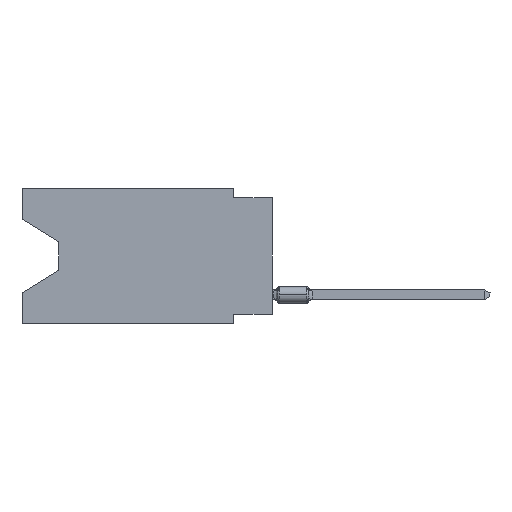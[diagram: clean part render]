
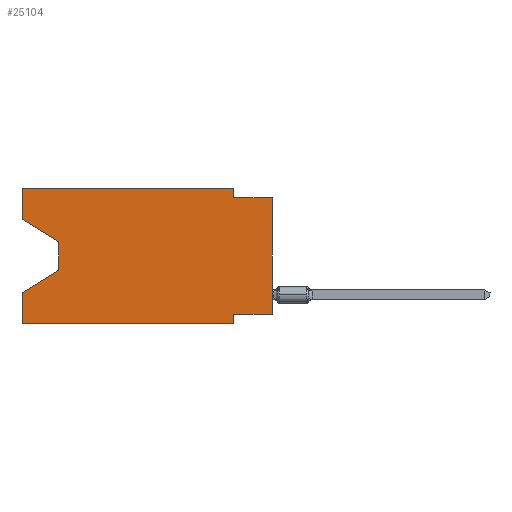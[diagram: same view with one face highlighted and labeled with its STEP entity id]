
A CAD part, left-side view. The second image highlights one B-rep face of the part: STEP entity #25104.
In plain terms, the highlighted planar face has unit normal (-1, 0, 0).
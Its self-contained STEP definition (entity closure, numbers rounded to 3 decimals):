
#1437 = VECTOR ( 'NONE', #28765, 1000. ) ;
#1544 = CARTESIAN_POINT ( 'NONE',  ( 0., 2.54, -0.635 ) ) ;
#2303 = CARTESIAN_POINT ( 'NONE',  ( 0., 2.54, -8.255 ) ) ;
#3989 = VECTOR ( 'NONE', #15168, 1000. ) ;
#4202 = VECTOR ( 'NONE', #17636, 1000. ) ;
#5450 = CARTESIAN_POINT ( 'NONE',  ( 0., 2.54, 0. ) ) ;
#5842 = VECTOR ( 'NONE', #18117, 1000. ) ;
#6163 = CARTESIAN_POINT ( 'NONE',  ( 0., 0., 0. ) ) ;
#6278 = VERTEX_POINT ( 'NONE', #1544 ) ;
#6721 = VERTEX_POINT ( 'NONE', #60788 ) ;
#7199 = EDGE_CURVE ( 'NONE', #6278, #15779, #60064, .T. ) ;
#8100 = ORIENTED_EDGE ( 'NONE', *, *, #58102, .T. ) ;
#9651 = VERTEX_POINT ( 'NONE', #30792 ) ;
#9822 = CARTESIAN_POINT ( 'NONE',  ( 0., 13.97, -3.505 ) ) ;
#9912 = ORIENTED_EDGE ( 'NONE', *, *, #25483, .T. ) ;
#10925 = LINE ( 'NONE', #55496, #21906 ) ;
#13155 = CARTESIAN_POINT ( 'NONE',  ( 0., 0., -0.635 ) ) ;
#14030 = CARTESIAN_POINT ( 'NONE',  ( 0., 13.97, -3.505 ) ) ;
#14526 = LINE ( 'NONE', #54491, #42638 ) ;
#14677 = DIRECTION ( 'NONE',  ( 0., 0., -1. ) ) ;
#15168 = DIRECTION ( 'NONE',  ( 0., -1., 0. ) ) ;
#15779 = VERTEX_POINT ( 'NONE', #13155 ) ;
#15805 = VERTEX_POINT ( 'NONE', #2303 ) ;
#17453 = CARTESIAN_POINT ( 'NONE',  ( 0., 13.97, -5.385 ) ) ;
#17636 = DIRECTION ( 'NONE',  ( 0., 0., 1. ) ) ;
#18117 = DIRECTION ( 'NONE',  ( 0., 0., -1. ) ) ;
#18408 = CARTESIAN_POINT ( 'NONE',  ( 0., 0., -8.255 ) ) ;
#19439 = DIRECTION ( 'NONE',  ( 0., -1., 0. ) ) ;
#20401 = VERTEX_POINT ( 'NONE', #29723 ) ;
#21127 = CARTESIAN_POINT ( 'NONE',  ( 0., 16.383, -6.852 ) ) ;
#21839 = VECTOR ( 'NONE', #31469, 1000. ) ;
#21906 = VECTOR ( 'NONE', #50893, 1000. ) ;
#22044 = LINE ( 'NONE', #17453, #44142 ) ;
#22450 = ORIENTED_EDGE ( 'NONE', *, *, #64841, .F. ) ;
#23852 = LINE ( 'NONE', #14030, #1437 ) ;
#23878 = VECTOR ( 'NONE', #45127, 1000. ) ;
#24247 = DIRECTION ( 'NONE',  ( 1., 0., 0. ) ) ;
#25104 = ADVANCED_FACE ( 'NONE', ( #58991 ), #54069, .F. ) ;
#25450 = EDGE_LOOP ( 'NONE', ( #8100, #9912, #36545, #36040, #64268, #38362, #22450, #37589, #34836, #39675, #56191, #43249 ) ) ;
#25483 = EDGE_CURVE ( 'NONE', #29320, #47591, #23852, .T. ) ;
#26862 = LINE ( 'NONE', #45880, #21839 ) ;
#27901 = EDGE_CURVE ( 'NONE', #46920, #57472, #14526, .T. ) ;
#28765 = DIRECTION ( 'NONE',  ( 0., 0., -1. ) ) ;
#29320 = VERTEX_POINT ( 'NONE', #9822 ) ;
#29723 = CARTESIAN_POINT ( 'NONE',  ( 0., 16.383, -2.038 ) ) ;
#30050 = EDGE_CURVE ( 'NONE', #20401, #31406, #10925, .T. ) ;
#30792 = CARTESIAN_POINT ( 'NONE',  ( 0., 0., -8.255 ) ) ;
#30953 = EDGE_CURVE ( 'NONE', #9651, #15779, #46144, .T. ) ;
#31406 = VERTEX_POINT ( 'NONE', #54150 ) ;
#31469 = DIRECTION ( 'NONE',  ( 0., -1., 0. ) ) ;
#34530 = CARTESIAN_POINT ( 'NONE',  ( 0., 0., -0.635 ) ) ;
#34752 = LINE ( 'NONE', #18408, #54293 ) ;
#34836 = ORIENTED_EDGE ( 'NONE', *, *, #7199, .F. ) ;
#35403 = VERTEX_POINT ( 'NONE', #63424 ) ;
#36040 = ORIENTED_EDGE ( 'NONE', *, *, #27901, .F. ) ;
#36545 = ORIENTED_EDGE ( 'NONE', *, *, #46083, .T. ) ;
#37589 = ORIENTED_EDGE ( 'NONE', *, *, #30953, .T. ) ;
#37802 = CARTESIAN_POINT ( 'NONE',  ( 0., 13.97, -5.385 ) ) ;
#38362 = ORIENTED_EDGE ( 'NONE', *, *, #53830, .F. ) ;
#38506 = AXIS2_PLACEMENT_3D ( 'NONE', #54712, #24247, #55026 ) ;
#38657 = EDGE_CURVE ( 'NONE', #35403, #6278, #55930, .T. ) ;
#39636 = VECTOR ( 'NONE', #19439, 1000. ) ;
#39675 = ORIENTED_EDGE ( 'NONE', *, *, #38657, .F. ) ;
#42027 = DIRECTION ( 'NONE',  ( 0., 0.855, -0.519 ) ) ;
#42502 = EDGE_CURVE ( 'NONE', #46920, #6721, #26862, .T. ) ;
#42638 = VECTOR ( 'NONE', #60360, 1000. ) ;
#43249 = ORIENTED_EDGE ( 'NONE', *, *, #30050, .F. ) ;
#43622 = DIRECTION ( 'NONE',  ( 0., 1., 0. ) ) ;
#44025 = LINE ( 'NONE', #44344, #39636 ) ;
#44142 = VECTOR ( 'NONE', #42027, 1000. ) ;
#44344 = CARTESIAN_POINT ( 'NONE',  ( 0., 16.383, 0. ) ) ;
#45127 = DIRECTION ( 'NONE',  ( 0., -0.855, -0.519 ) ) ;
#45880 = CARTESIAN_POINT ( 'NONE',  ( 0., 16.383, -8.89 ) ) ;
#46083 = EDGE_CURVE ( 'NONE', #47591, #57472, #22044, .T. ) ;
#46144 = LINE ( 'NONE', #6163, #4202 ) ;
#46920 = VERTEX_POINT ( 'NONE', #48016 ) ;
#47591 = VERTEX_POINT ( 'NONE', #37802 ) ;
#48016 = CARTESIAN_POINT ( 'NONE',  ( 0., 16.383, -8.89 ) ) ;
#48253 = CARTESIAN_POINT ( 'NONE',  ( 0., 2.54, -8.89 ) ) ;
#50893 = DIRECTION ( 'NONE',  ( 0., 0., 1. ) ) ;
#53830 = EDGE_CURVE ( 'NONE', #15805, #6721, #57449, .T. ) ;
#54069 = PLANE ( 'NONE',  #38506 ) ;
#54150 = CARTESIAN_POINT ( 'NONE',  ( 0., 16.383, 0. ) ) ;
#54293 = VECTOR ( 'NONE', #43622, 1000. ) ;
#54491 = CARTESIAN_POINT ( 'NONE',  ( 0., 16.383, 0. ) ) ;
#54712 = CARTESIAN_POINT ( 'NONE',  ( 0., 16.383, 0. ) ) ;
#55026 = DIRECTION ( 'NONE',  ( 0., 0., -1. ) ) ;
#55496 = CARTESIAN_POINT ( 'NONE',  ( 0., 16.383, 0. ) ) ;
#55930 = LINE ( 'NONE', #5450, #63308 ) ;
#55944 = CARTESIAN_POINT ( 'NONE',  ( 0., 16.383, -2.038 ) ) ;
#56191 = ORIENTED_EDGE ( 'NONE', *, *, #64464, .F. ) ;
#57449 = LINE ( 'NONE', #48253, #5842 ) ;
#57472 = VERTEX_POINT ( 'NONE', #21127 ) ;
#58102 = EDGE_CURVE ( 'NONE', #20401, #29320, #60215, .T. ) ;
#58991 = FACE_OUTER_BOUND ( 'NONE', #25450, .T. ) ;
#60064 = LINE ( 'NONE', #34530, #3989 ) ;
#60215 = LINE ( 'NONE', #55944, #23878 ) ;
#60360 = DIRECTION ( 'NONE',  ( 0., 0., 1. ) ) ;
#60788 = CARTESIAN_POINT ( 'NONE',  ( 0., 2.54, -8.89 ) ) ;
#63308 = VECTOR ( 'NONE', #14677, 1000. ) ;
#63424 = CARTESIAN_POINT ( 'NONE',  ( 0., 2.54, 0. ) ) ;
#64268 = ORIENTED_EDGE ( 'NONE', *, *, #42502, .T. ) ;
#64464 = EDGE_CURVE ( 'NONE', #31406, #35403, #44025, .T. ) ;
#64841 = EDGE_CURVE ( 'NONE', #9651, #15805, #34752, .T. ) ;
